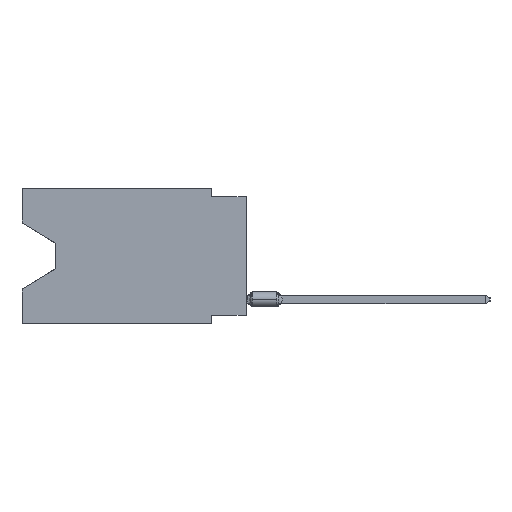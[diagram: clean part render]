
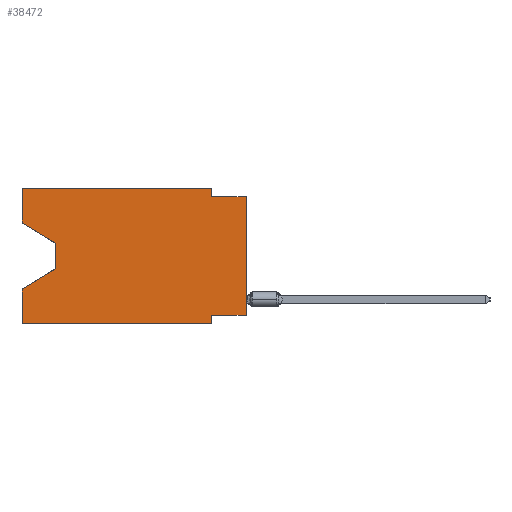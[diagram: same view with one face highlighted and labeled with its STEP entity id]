
A CAD part, left-side view. The second image highlights one B-rep face of the part: STEP entity #38472.
In plain terms, the highlighted planar face has unit normal (-1, 0, 0).
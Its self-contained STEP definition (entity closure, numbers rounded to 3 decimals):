
#44 = CARTESIAN_POINT ( 'NONE',  ( 0., 16.383, -2.546 ) ) ;
#2925 = CARTESIAN_POINT ( 'NONE',  ( 0., 0., -0.635 ) ) ;
#3054 = LINE ( 'NONE', #13350, #45913 ) ;
#3067 = ORIENTED_EDGE ( 'NONE', *, *, #8241, .T. ) ;
#3074 = PLANE ( 'NONE',  #21290 ) ;
#3164 = DIRECTION ( 'NONE',  ( 0., -1., 0. ) ) ;
#3381 = ORIENTED_EDGE ( 'NONE', *, *, #6472, .T. ) ;
#3731 = ORIENTED_EDGE ( 'NONE', *, *, #31776, .F. ) ;
#3787 = CARTESIAN_POINT ( 'NONE',  ( 0., 13.97, -4.013 ) ) ;
#4040 = EDGE_LOOP ( 'NONE', ( #6492, #3381, #3067, #19882, #14014, #14942, #32487, #17632, #18193, #10692, #3731, #14159 ) ) ;
#4608 = VECTOR ( 'NONE', #11957, 1000. ) ;
#4799 = DIRECTION ( 'NONE',  ( 0., 1., 0. ) ) ;
#4986 = VERTEX_POINT ( 'NONE', #35504 ) ;
#5027 = VECTOR ( 'NONE', #3164, 1000. ) ;
#5040 = CARTESIAN_POINT ( 'NONE',  ( 0., 0., -9.271 ) ) ;
#6443 = VERTEX_POINT ( 'NONE', #21523 ) ;
#6472 = EDGE_CURVE ( 'NONE', #28337, #43929, #30101, .T. ) ;
#6492 = ORIENTED_EDGE ( 'NONE', *, *, #21017, .T. ) ;
#7063 = LINE ( 'NONE', #2925, #5027 ) ;
#7748 = CARTESIAN_POINT ( 'NONE',  ( 0., 2.54, -0.635 ) ) ;
#8241 = EDGE_CURVE ( 'NONE', #43929, #27168, #40526, .T. ) ;
#8537 = VECTOR ( 'NONE', #20256, 1000. ) ;
#8895 = LINE ( 'NONE', #20175, #24900 ) ;
#9336 = VECTOR ( 'NONE', #41777, 1000. ) ;
#9919 = DIRECTION ( 'NONE',  ( 1., 0., 0. ) ) ;
#10128 = DIRECTION ( 'NONE',  ( 0., 0.855, -0.519 ) ) ;
#10692 = ORIENTED_EDGE ( 'NONE', *, *, #23345, .F. ) ;
#11078 = VERTEX_POINT ( 'NONE', #46482 ) ;
#11506 = VERTEX_POINT ( 'NONE', #46601 ) ;
#11754 = VECTOR ( 'NONE', #15076, 1000. ) ;
#11957 = DIRECTION ( 'NONE',  ( 0., 0., -1. ) ) ;
#12027 = EDGE_CURVE ( 'NONE', #42126, #23524, #7063, .T. ) ;
#13350 = CARTESIAN_POINT ( 'NONE',  ( 0., 16.383, 0. ) ) ;
#13648 = DIRECTION ( 'NONE',  ( 0., 0., 1. ) ) ;
#14014 = ORIENTED_EDGE ( 'NONE', *, *, #15356, .T. ) ;
#14159 = ORIENTED_EDGE ( 'NONE', *, *, #26851, .F. ) ;
#14683 = VERTEX_POINT ( 'NONE', #41681 ) ;
#14942 = ORIENTED_EDGE ( 'NONE', *, *, #20512, .F. ) ;
#15076 = DIRECTION ( 'NONE',  ( 0., -1., 0. ) ) ;
#15356 = EDGE_CURVE ( 'NONE', #6443, #4986, #26780, .T. ) ;
#15794 = CARTESIAN_POINT ( 'NONE',  ( 0., 16.383, -2.546 ) ) ;
#16478 = DIRECTION ( 'NONE',  ( 0., -1., 0. ) ) ;
#17369 = CARTESIAN_POINT ( 'NONE',  ( 0., 13.97, -5.893 ) ) ;
#17632 = ORIENTED_EDGE ( 'NONE', *, *, #18992, .T. ) ;
#18193 = ORIENTED_EDGE ( 'NONE', *, *, #12027, .F. ) ;
#18992 = EDGE_CURVE ( 'NONE', #11078, #23524, #8895, .T. ) ;
#19882 = ORIENTED_EDGE ( 'NONE', *, *, #26465, .F. ) ;
#20175 = CARTESIAN_POINT ( 'NONE',  ( 0., 0., 0. ) ) ;
#20256 = DIRECTION ( 'NONE',  ( 0., 0., -1. ) ) ;
#20512 = EDGE_CURVE ( 'NONE', #14683, #4986, #39134, .T. ) ;
#20811 = CARTESIAN_POINT ( 'NONE',  ( 0., 16.383, -7.36 ) ) ;
#21017 = EDGE_CURVE ( 'NONE', #24617, #28337, #35125, .T. ) ;
#21290 = AXIS2_PLACEMENT_3D ( 'NONE', #43498, #9919, #32945 ) ;
#21463 = CARTESIAN_POINT ( 'NONE',  ( 0., 16.383, 0. ) ) ;
#21523 = CARTESIAN_POINT ( 'NONE',  ( 0., 16.383, -9.906 ) ) ;
#23345 = EDGE_CURVE ( 'NONE', #11506, #42126, #42025, .T. ) ;
#23524 = VERTEX_POINT ( 'NONE', #47876 ) ;
#24271 = VECTOR ( 'NONE', #4799, 1000. ) ;
#24617 = VERTEX_POINT ( 'NONE', #44 ) ;
#24900 = VECTOR ( 'NONE', #35106, 1000. ) ;
#25026 = VERTEX_POINT ( 'NONE', #25686 ) ;
#25505 = VECTOR ( 'NONE', #13648, 1000. ) ;
#25686 = CARTESIAN_POINT ( 'NONE',  ( 0., 16.383, 0. ) ) ;
#26465 = EDGE_CURVE ( 'NONE', #6443, #27168, #28588, .T. ) ;
#26780 = LINE ( 'NONE', #30924, #30989 ) ;
#26851 = EDGE_CURVE ( 'NONE', #24617, #25026, #3054, .T. ) ;
#27168 = VERTEX_POINT ( 'NONE', #20811 ) ;
#28210 = VECTOR ( 'NONE', #10128, 1000. ) ;
#28337 = VERTEX_POINT ( 'NONE', #3787 ) ;
#28552 = FACE_OUTER_BOUND ( 'NONE', #4040, .T. ) ;
#28588 = LINE ( 'NONE', #21463, #25505 ) ;
#29111 = LINE ( 'NONE', #43577, #11754 ) ;
#30101 = LINE ( 'NONE', #41629, #4608 ) ;
#30924 = CARTESIAN_POINT ( 'NONE',  ( 0., 16.383, -9.906 ) ) ;
#30989 = VECTOR ( 'NONE', #16478, 1000. ) ;
#31776 = EDGE_CURVE ( 'NONE', #25026, #11506, #29111, .T. ) ;
#31956 = CARTESIAN_POINT ( 'NONE',  ( 0., 2.54, 0. ) ) ;
#32299 = VECTOR ( 'NONE', #45945, 1000. ) ;
#32487 = ORIENTED_EDGE ( 'NONE', *, *, #48130, .F. ) ;
#32945 = DIRECTION ( 'NONE',  ( 0., 0., -1. ) ) ;
#35106 = DIRECTION ( 'NONE',  ( 0., 0., 1. ) ) ;
#35125 = LINE ( 'NONE', #15794, #9336 ) ;
#35504 = CARTESIAN_POINT ( 'NONE',  ( 0., 2.54, -9.906 ) ) ;
#38472 = ADVANCED_FACE ( 'NONE', ( #28552 ), #3074, .F. ) ;
#39134 = LINE ( 'NONE', #43043, #8537 ) ;
#40526 = LINE ( 'NONE', #40773, #28210 ) ;
#40773 = CARTESIAN_POINT ( 'NONE',  ( 0., 13.97, -5.893 ) ) ;
#41629 = CARTESIAN_POINT ( 'NONE',  ( 0., 13.97, -4.013 ) ) ;
#41681 = CARTESIAN_POINT ( 'NONE',  ( 0., 2.54, -9.271 ) ) ;
#41777 = DIRECTION ( 'NONE',  ( 0., -0.855, -0.519 ) ) ;
#42025 = LINE ( 'NONE', #31956, #32299 ) ;
#42126 = VERTEX_POINT ( 'NONE', #7748 ) ;
#42287 = LINE ( 'NONE', #5040, #24271 ) ;
#43043 = CARTESIAN_POINT ( 'NONE',  ( 0., 2.54, -9.906 ) ) ;
#43481 = DIRECTION ( 'NONE',  ( 0., 0., 1. ) ) ;
#43498 = CARTESIAN_POINT ( 'NONE',  ( 0., 16.383, 0. ) ) ;
#43577 = CARTESIAN_POINT ( 'NONE',  ( 0., 16.383, 0. ) ) ;
#43929 = VERTEX_POINT ( 'NONE', #17369 ) ;
#45913 = VECTOR ( 'NONE', #43481, 1000. ) ;
#45945 = DIRECTION ( 'NONE',  ( 0., 0., -1. ) ) ;
#46482 = CARTESIAN_POINT ( 'NONE',  ( 0., 0., -9.271 ) ) ;
#46601 = CARTESIAN_POINT ( 'NONE',  ( 0., 2.54, 0. ) ) ;
#47876 = CARTESIAN_POINT ( 'NONE',  ( 0., 0., -0.635 ) ) ;
#48130 = EDGE_CURVE ( 'NONE', #11078, #14683, #42287, .T. ) ;
